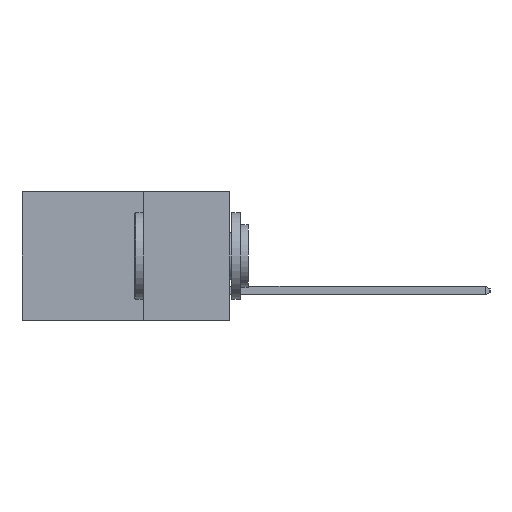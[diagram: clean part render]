
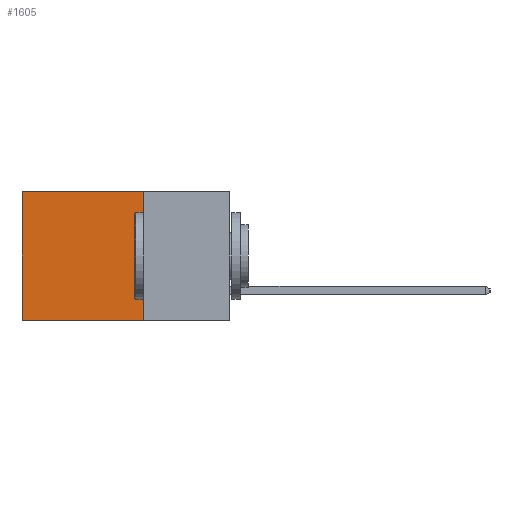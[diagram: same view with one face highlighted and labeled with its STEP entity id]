
A CAD part, left-side view. The second image highlights one B-rep face of the part: STEP entity #1605.
In plain terms, the highlighted planar face has unit normal (-1, 0, 0).
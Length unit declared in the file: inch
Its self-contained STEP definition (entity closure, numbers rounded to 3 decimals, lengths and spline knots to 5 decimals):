
#396 = FACE_OUTER_BOUND ( 'NONE', #4615, .T. ) ;
#842 = EDGE_CURVE ( 'NONE', #10570, #1998, #8749, .T. ) ;
#1208 = LINE ( 'NONE', #13072, #15644 ) ;
#1605 = ADVANCED_FACE ( 'NONE', ( #396 ), #10308, .F. ) ;
#1998 = VERTEX_POINT ( 'NONE', #8619 ) ;
#2490 = ORIENTED_EDGE ( 'NONE', *, *, #14555, .T. ) ;
#3737 = EDGE_CURVE ( 'NONE', #11289, #10570, #7502, .T. ) ;
#4095 = DIRECTION ( 'NONE',  ( 0., 0., -1. ) ) ;
#4615 = EDGE_LOOP ( 'NONE', ( #2490, #8273, #14955, #19140 ) ) ;
#5341 = CARTESIAN_POINT ( 'NONE',  ( 0.298, 0.6, 0. ) ) ;
#5970 = CARTESIAN_POINT ( 'NONE',  ( 0.298, 0.25, 0. ) ) ;
#6357 = VECTOR ( 'NONE', #4095, 39.37008 ) ;
#6897 = VECTOR ( 'NONE', #19483, 39.37008 ) ;
#7502 = LINE ( 'NONE', #5970, #6897 ) ;
#7757 = CARTESIAN_POINT ( 'NONE',  ( 0.298, 0.25, 0. ) ) ;
#8273 = ORIENTED_EDGE ( 'NONE', *, *, #842, .F. ) ;
#8619 = CARTESIAN_POINT ( 'NONE',  ( 0.298, 0.6, -0.37 ) ) ;
#8749 = LINE ( 'NONE', #17343, #22517 ) ;
#10021 = DIRECTION ( 'NONE',  ( 1., 0., 0. ) ) ;
#10308 = PLANE ( 'NONE',  #11241 ) ;
#10570 = VERTEX_POINT ( 'NONE', #20447 ) ;
#11189 = DIRECTION ( 'NONE',  ( 0., 1., 0. ) ) ;
#11241 = AXIS2_PLACEMENT_3D ( 'NONE', #7757, #10021, #21474 ) ;
#11289 = VERTEX_POINT ( 'NONE', #20829 ) ;
#13072 = CARTESIAN_POINT ( 'NONE',  ( 0.298, 0.25, 0. ) ) ;
#14555 = EDGE_CURVE ( 'NONE', #17822, #1998, #21980, .T. ) ;
#14955 = ORIENTED_EDGE ( 'NONE', *, *, #3737, .F. ) ;
#15644 = VECTOR ( 'NONE', #11189, 39.37008 ) ;
#16643 = EDGE_CURVE ( 'NONE', #11289, #17822, #1208, .T. ) ;
#17288 = CARTESIAN_POINT ( 'NONE',  ( 0.298, 0.6, 0. ) ) ;
#17343 = CARTESIAN_POINT ( 'NONE',  ( 0.298, 0.25, -0.37 ) ) ;
#17822 = VERTEX_POINT ( 'NONE', #5341 ) ;
#17839 = DIRECTION ( 'NONE',  ( 0., 1., 0. ) ) ;
#19140 = ORIENTED_EDGE ( 'NONE', *, *, #16643, .T. ) ;
#19483 = DIRECTION ( 'NONE',  ( 0., 0., -1. ) ) ;
#20447 = CARTESIAN_POINT ( 'NONE',  ( 0.298, 0.25, -0.37 ) ) ;
#20829 = CARTESIAN_POINT ( 'NONE',  ( 0.298, 0.25, 0. ) ) ;
#21474 = DIRECTION ( 'NONE',  ( 0., 0., -1. ) ) ;
#21980 = LINE ( 'NONE', #17288, #6357 ) ;
#22517 = VECTOR ( 'NONE', #17839, 39.37008 ) ;
